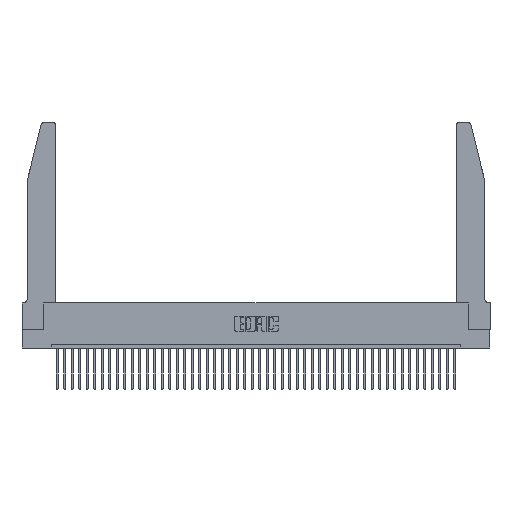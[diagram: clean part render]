
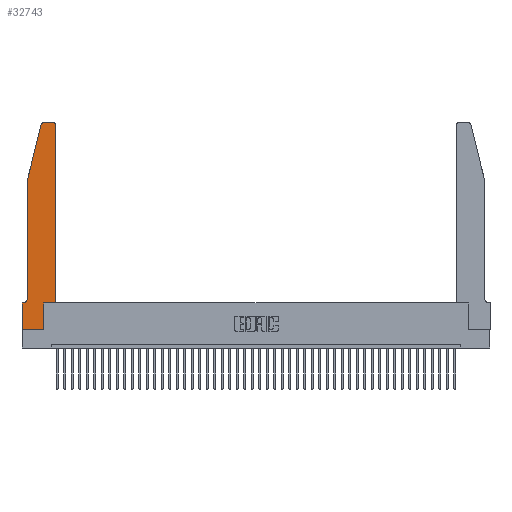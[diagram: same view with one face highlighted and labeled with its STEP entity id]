
A CAD part, top view. The second image highlights one B-rep face of the part: STEP entity #32743.
In plain terms, the highlighted planar face has unit normal (0, 0, 1).
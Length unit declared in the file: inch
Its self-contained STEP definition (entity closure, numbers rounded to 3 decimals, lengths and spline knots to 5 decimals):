
#71 = DIRECTION ( 'NONE',  ( 1., 0., 0. ) ) ;
#325 = DIRECTION ( 'NONE',  ( -1., 0., 0. ) ) ;
#920 = VECTOR ( 'NONE', #27111, 39.37008 ) ;
#1531 = CARTESIAN_POINT ( 'NONE',  ( 0.4505, 0.35, 0.37 ) ) ;
#1633 = ORIENTED_EDGE ( 'NONE', *, *, #27751, .T. ) ;
#1751 = VECTOR ( 'NONE', #8812, 39.37008 ) ;
#2116 = CARTESIAN_POINT ( 'NONE',  ( 0.0755, 2., 0.37 ) ) ;
#2885 = EDGE_CURVE ( 'NONE', #29325, #30106, #29284, .T. ) ;
#3393 = CARTESIAN_POINT ( 'NONE',  ( 0., 0., 0.37 ) ) ;
#3635 = CARTESIAN_POINT ( 'NONE',  ( 0.0055, 0.35, 0.37 ) ) ;
#4388 = LINE ( 'NONE', #35248, #15731 ) ;
#4609 = VERTEX_POINT ( 'NONE', #35180 ) ;
#4719 = DIRECTION ( 'NONE',  ( 0., 0., 1. ) ) ;
#5474 = CARTESIAN_POINT ( 'NONE',  ( 0., 0., 0.37 ) ) ;
#5608 = ORIENTED_EDGE ( 'NONE', *, *, #35184, .T. ) ;
#5615 = VERTEX_POINT ( 'NONE', #12916 ) ;
#5626 = DIRECTION ( 'NONE',  ( 0., 0., 1. ) ) ;
#6385 = CARTESIAN_POINT ( 'NONE',  ( 0.0755, 2., 0.37 ) ) ;
#7269 = EDGE_LOOP ( 'NONE', ( #12412, #27801, #8535, #8686, #17887, #1633, #5608, #35289, #13031, #28746, #10041, #26654 ) ) ;
#7375 = FACE_OUTER_BOUND ( 'NONE', #7269, .T. ) ;
#7508 = CARTESIAN_POINT ( 'NONE',  ( 0.0755, 2., 0.37 ) ) ;
#7919 = VERTEX_POINT ( 'NONE', #38720 ) ;
#8215 = VECTOR ( 'NONE', #12143, 39.37008 ) ;
#8311 = DIRECTION ( 'NONE',  ( -1., 0., 0. ) ) ;
#8535 = ORIENTED_EDGE ( 'NONE', *, *, #2885, .T. ) ;
#8686 = ORIENTED_EDGE ( 'NONE', *, *, #17607, .T. ) ;
#8812 = DIRECTION ( 'NONE',  ( -0.239, -0.971, 0. ) ) ;
#8921 = VERTEX_POINT ( 'NONE', #38659 ) ;
#9738 = VECTOR ( 'NONE', #8311, 39.37008 ) ;
#9958 = CARTESIAN_POINT ( 'NONE',  ( 0.25487, 2.72718, 0.37 ) ) ;
#10041 = ORIENTED_EDGE ( 'NONE', *, *, #21792, .T. ) ;
#10595 = VERTEX_POINT ( 'NONE', #33971 ) ;
#11373 = DIRECTION ( 'NONE',  ( 0., -1., 0. ) ) ;
#11539 = DIRECTION ( 'NONE',  ( 1., 0., 0. ) ) ;
#11549 = CARTESIAN_POINT ( 'NONE',  ( 0.284, 2.72, 0.37 ) ) ;
#12143 = DIRECTION ( 'NONE',  ( 0., -1., 0. ) ) ;
#12412 = ORIENTED_EDGE ( 'NONE', *, *, #17539, .T. ) ;
#12916 = CARTESIAN_POINT ( 'NONE',  ( 0.0755, 0.42, 0.37 ) ) ;
#12984 = VERTEX_POINT ( 'NONE', #21638 ) ;
#13031 = ORIENTED_EDGE ( 'NONE', *, *, #23760, .T. ) ;
#13580 = VECTOR ( 'NONE', #32184, 39.37008 ) ;
#13824 = CARTESIAN_POINT ( 'NONE',  ( 0.0755, 0.35, 0.37 ) ) ;
#14629 = DIRECTION ( 'NONE',  ( 1., 0., 0. ) ) ;
#14953 = DIRECTION ( 'NONE',  ( 0., 1., 0. ) ) ;
#15255 = CARTESIAN_POINT ( 'NONE',  ( 0.2865, 0.35, 0.37 ) ) ;
#15731 = VECTOR ( 'NONE', #14953, 39.37008 ) ;
#17086 = EDGE_CURVE ( 'NONE', #8921, #29325, #39396, .T. ) ;
#17123 = LINE ( 'NONE', #6385, #40503 ) ;
#17539 = EDGE_CURVE ( 'NONE', #10595, #8921, #18786, .T. ) ;
#17607 = EDGE_CURVE ( 'NONE', #30106, #5615, #17123, .T. ) ;
#17887 = ORIENTED_EDGE ( 'NONE', *, *, #34767, .T. ) ;
#18408 = CARTESIAN_POINT ( 'NONE',  ( 0.4505, 2.72, 0.37 ) ) ;
#18786 = LINE ( 'NONE', #30576, #9738 ) ;
#20088 = VERTEX_POINT ( 'NONE', #5474 ) ;
#20284 = EDGE_CURVE ( 'NONE', #21600, #7919, #37567, .T. ) ;
#21600 = VERTEX_POINT ( 'NONE', #15255 ) ;
#21638 = CARTESIAN_POINT ( 'NONE',  ( 0., 0.35, 0.37 ) ) ;
#21792 = EDGE_CURVE ( 'NONE', #7919, #25943, #30569, .T. ) ;
#23760 = EDGE_CURVE ( 'NONE', #4609, #21600, #4388, .T. ) ;
#25943 = VERTEX_POINT ( 'NONE', #18408 ) ;
#25946 = CARTESIAN_POINT ( 'NONE',  ( 0.4205, 2.72, 0.37 ) ) ;
#26004 = AXIS2_PLACEMENT_3D ( 'NONE', #11549, #4719, #14629 ) ;
#26654 = ORIENTED_EDGE ( 'NONE', *, *, #36862, .T. ) ;
#26928 = VERTEX_POINT ( 'NONE', #3635 ) ;
#27111 = DIRECTION ( 'NONE',  ( 1., 0., 0. ) ) ;
#27751 = EDGE_CURVE ( 'NONE', #26928, #12984, #30222, .T. ) ;
#27801 = ORIENTED_EDGE ( 'NONE', *, *, #17086, .T. ) ;
#28372 = PLANE ( 'NONE',  #36297 ) ;
#28746 = ORIENTED_EDGE ( 'NONE', *, *, #20284, .T. ) ;
#29284 = LINE ( 'NONE', #2116, #1751 ) ;
#29325 = VERTEX_POINT ( 'NONE', #9958 ) ;
#30106 = VERTEX_POINT ( 'NONE', #7508 ) ;
#30222 = LINE ( 'NONE', #13824, #38654 ) ;
#30569 = LINE ( 'NONE', #1531, #13580 ) ;
#30576 = CARTESIAN_POINT ( 'NONE',  ( 0.2605, 2.75, 0.37 ) ) ;
#31779 = DIRECTION ( 'NONE',  ( 1., 0., 0. ) ) ;
#32143 = LINE ( 'NONE', #35535, #8215 ) ;
#32184 = DIRECTION ( 'NONE',  ( 0., 1., 0. ) ) ;
#32743 = ADVANCED_FACE ( 'NONE', ( #7375 ), #28372, .T. ) ;
#32960 = DIRECTION ( 'NONE',  ( 0., 0., -1. ) ) ;
#33971 = CARTESIAN_POINT ( 'NONE',  ( 0.4205, 2.75, 0.37 ) ) ;
#34715 = EDGE_CURVE ( 'NONE', #20088, #4609, #34769, .T. ) ;
#34767 = EDGE_CURVE ( 'NONE', #5615, #26928, #35888, .T. ) ;
#34769 = LINE ( 'NONE', #3393, #920 ) ;
#34967 = CARTESIAN_POINT ( 'NONE',  ( 0., 0.35, 0.37 ) ) ;
#35180 = CARTESIAN_POINT ( 'NONE',  ( 0.2865, 0., 0.37 ) ) ;
#35184 = EDGE_CURVE ( 'NONE', #12984, #20088, #32143, .T. ) ;
#35248 = CARTESIAN_POINT ( 'NONE',  ( 0.2865, 0.35, 0.37 ) ) ;
#35289 = ORIENTED_EDGE ( 'NONE', *, *, #34715, .T. ) ;
#35535 = CARTESIAN_POINT ( 'NONE',  ( 0., 0., 0.37 ) ) ;
#35888 = CIRCLE ( 'NONE', #39766, 0.07 ) ;
#36297 = AXIS2_PLACEMENT_3D ( 'NONE', #34967, #38364, #31779 ) ;
#36862 = EDGE_CURVE ( 'NONE', #25943, #10595, #39897, .T. ) ;
#37507 = DIRECTION ( 'NONE',  ( -1., 0., 0. ) ) ;
#37567 = LINE ( 'NONE', #42060, #41289 ) ;
#38364 = DIRECTION ( 'NONE',  ( 0., 0., 1. ) ) ;
#38654 = VECTOR ( 'NONE', #37507, 39.37008 ) ;
#38659 = CARTESIAN_POINT ( 'NONE',  ( 0.284, 2.75, 0.37 ) ) ;
#38720 = CARTESIAN_POINT ( 'NONE',  ( 0.4505, 0.35, 0.37 ) ) ;
#39396 = CIRCLE ( 'NONE', #26004, 0.03 ) ;
#39766 = AXIS2_PLACEMENT_3D ( 'NONE', #41365, #32960, #325 ) ;
#39897 = CIRCLE ( 'NONE', #39980, 0.03 ) ;
#39980 = AXIS2_PLACEMENT_3D ( 'NONE', #25946, #5626, #71 ) ;
#40503 = VECTOR ( 'NONE', #11373, 39.37008 ) ;
#41289 = VECTOR ( 'NONE', #11539, 39.37008 ) ;
#41365 = CARTESIAN_POINT ( 'NONE',  ( 0.0055, 0.42, 0.37 ) ) ;
#42060 = CARTESIAN_POINT ( 'NONE',  ( 0.4505, 0.35, 0.37 ) ) ;
